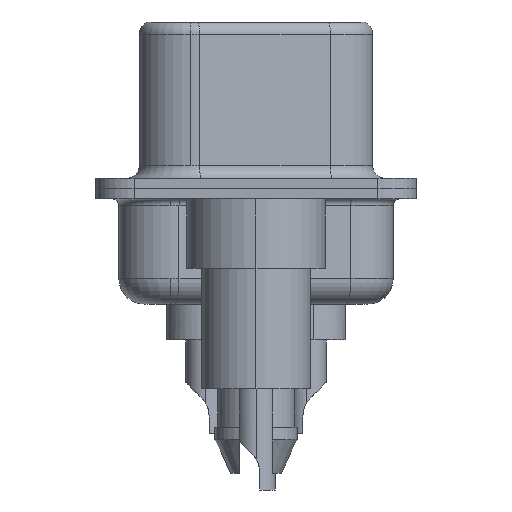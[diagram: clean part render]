
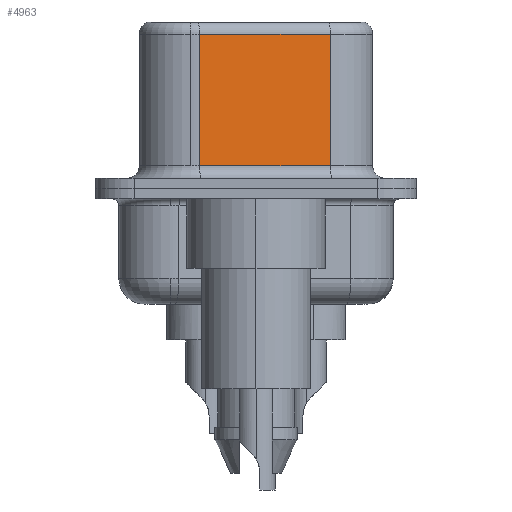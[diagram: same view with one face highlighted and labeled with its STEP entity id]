
A CAD part, left-side view. The second image highlights one B-rep face of the part: STEP entity #4963.
In plain terms, the highlighted planar face has unit normal (-0.985, -0.174, 0).
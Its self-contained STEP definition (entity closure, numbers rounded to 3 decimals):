
#1250 = ORIENTED_EDGE ( 'NONE', *, *, #4157, .T. ) ;
#1476 = LINE ( 'NONE', #4104, #18873 ) ;
#2294 = DIRECTION ( 'NONE',  ( 0., 0., -1. ) ) ;
#2761 = VERTEX_POINT ( 'NONE', #5573 ) ;
#4104 = CARTESIAN_POINT ( 'NONE',  ( 4.555, -2.897, 6.02 ) ) ;
#4157 = EDGE_CURVE ( 'NONE', #2761, #12281, #7350, .T. ) ;
#4178 = DIRECTION ( 'NONE',  ( -0.174, 0.985, 0. ) ) ;
#4561 = ORIENTED_EDGE ( 'NONE', *, *, #14144, .T. ) ;
#4730 = EDGE_CURVE ( 'NONE', #14832, #12281, #19526, .T. ) ;
#4963 = ADVANCED_FACE ( 'NONE', ( #16457 ), #18406, .F. ) ;
#5573 = CARTESIAN_POINT ( 'NONE',  ( 3.655, 2.203, 0.9 ) ) ;
#5773 = CARTESIAN_POINT ( 'NONE',  ( 3.655, 2.203, 6.52 ) ) ;
#6044 = VECTOR ( 'NONE', #2294, 1000. ) ;
#6052 = CARTESIAN_POINT ( 'NONE',  ( 4.555, -2.897, 0.9 ) ) ;
#6495 = DIRECTION ( 'NONE',  ( 0.174, -0.985, 0. ) ) ;
#7350 = LINE ( 'NONE', #6052, #14733 ) ;
#7522 = CARTESIAN_POINT ( 'NONE',  ( 4.555, -2.897, 0.9 ) ) ;
#10055 = DIRECTION ( 'NONE',  ( 0., 0., -1. ) ) ;
#10202 = CARTESIAN_POINT ( 'NONE',  ( 4.555, -2.897, 6.52 ) ) ;
#10458 = VERTEX_POINT ( 'NONE', #11507 ) ;
#11249 = ORIENTED_EDGE ( 'NONE', *, *, #4730, .F. ) ;
#11507 = CARTESIAN_POINT ( 'NONE',  ( 3.655, 2.203, 6.02 ) ) ;
#12200 = ORIENTED_EDGE ( 'NONE', *, *, #17636, .T. ) ;
#12281 = VERTEX_POINT ( 'NONE', #7522 ) ;
#14144 = EDGE_CURVE ( 'NONE', #10458, #2761, #15020, .T. ) ;
#14479 = EDGE_LOOP ( 'NONE', ( #11249, #12200, #4561, #1250 ) ) ;
#14733 = VECTOR ( 'NONE', #6495, 1000. ) ;
#14832 = VERTEX_POINT ( 'NONE', #17399 ) ;
#15020 = LINE ( 'NONE', #5773, #6044 ) ;
#16457 = FACE_OUTER_BOUND ( 'NONE', #14479, .T. ) ;
#16715 = VECTOR ( 'NONE', #10055, 1000. ) ;
#17399 = CARTESIAN_POINT ( 'NONE',  ( 4.555, -2.897, 6.02 ) ) ;
#17636 = EDGE_CURVE ( 'NONE', #14832, #10458, #1476, .T. ) ;
#18240 = DIRECTION ( 'NONE',  ( -0.174, 0.985, 0. ) ) ;
#18320 = DIRECTION ( 'NONE',  ( 0.985, 0.174, 0. ) ) ;
#18402 = CARTESIAN_POINT ( 'NONE',  ( 4.555, -2.897, 6.52 ) ) ;
#18406 = PLANE ( 'NONE',  #20782 ) ;
#18873 = VECTOR ( 'NONE', #4178, 1000. ) ;
#19526 = LINE ( 'NONE', #10202, #16715 ) ;
#20782 = AXIS2_PLACEMENT_3D ( 'NONE', #18402, #18320, #18240 ) ;
